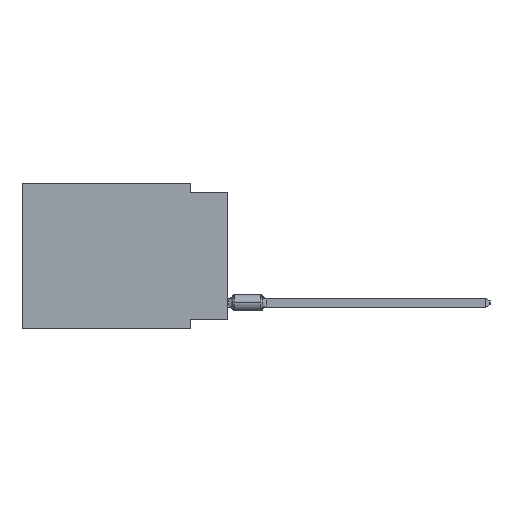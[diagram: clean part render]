
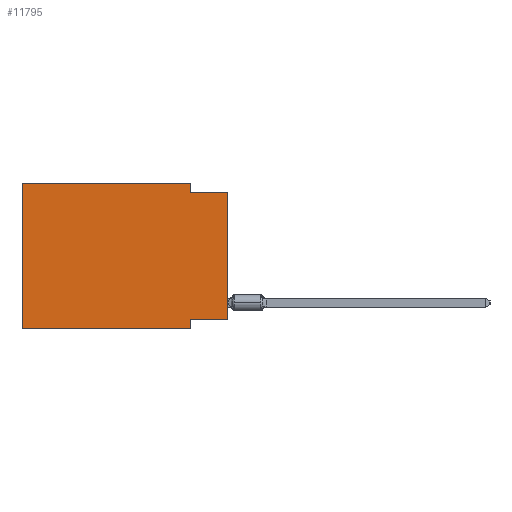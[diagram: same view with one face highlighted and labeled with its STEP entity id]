
A CAD part, left-side view. The second image highlights one B-rep face of the part: STEP entity #11795.
In plain terms, the highlighted planar face has unit normal (-1, 0, 0).
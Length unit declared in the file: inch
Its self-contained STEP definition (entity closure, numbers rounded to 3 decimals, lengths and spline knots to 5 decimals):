
#186 = VECTOR ( 'NONE', #24323, 39.37008 ) ;
#925 = ORIENTED_EDGE ( 'NONE', *, *, #29303, .F. ) ;
#1078 = DIRECTION ( 'NONE',  ( 0., 0., 1. ) ) ;
#1138 = VERTEX_POINT ( 'NONE', #26787 ) ;
#2114 = EDGE_CURVE ( 'NONE', #17205, #2430, #9782, .T. ) ;
#2336 = CARTESIAN_POINT ( 'NONE',  ( 0., 0.1, -0.365 ) ) ;
#2430 = VERTEX_POINT ( 'NONE', #2944 ) ;
#2562 = ORIENTED_EDGE ( 'NONE', *, *, #2114, .T. ) ;
#2828 = DIRECTION ( 'NONE',  ( 0., 1., 0. ) ) ;
#2858 = CARTESIAN_POINT ( 'NONE',  ( 0., 0.1, 0. ) ) ;
#2944 = CARTESIAN_POINT ( 'NONE',  ( 0., 0., -0.025 ) ) ;
#3008 = CARTESIAN_POINT ( 'NONE',  ( 0., 0., -0.365 ) ) ;
#3249 = DIRECTION ( 'NONE',  ( 0., 0., -1. ) ) ;
#4043 = LINE ( 'NONE', #18468, #186 ) ;
#4819 = CARTESIAN_POINT ( 'NONE',  ( 0., 0.55, -0.39 ) ) ;
#6089 = EDGE_CURVE ( 'NONE', #13038, #1138, #30358, .T. ) ;
#8978 = DIRECTION ( 'NONE',  ( 0., -1., 0. ) ) ;
#9512 = VERTEX_POINT ( 'NONE', #4819 ) ;
#9751 = EDGE_CURVE ( 'NONE', #30441, #13185, #4043, .T. ) ;
#9782 = LINE ( 'NONE', #32372, #20510 ) ;
#10248 = CARTESIAN_POINT ( 'NONE',  ( 0., 0.1, 0. ) ) ;
#11617 = CARTESIAN_POINT ( 'NONE',  ( 0., 0., -0.025 ) ) ;
#11773 = PLANE ( 'NONE',  #33305 ) ;
#11795 = ADVANCED_FACE ( 'NONE', ( #17851 ), #11773, .F. ) ;
#11846 = LINE ( 'NONE', #23409, #24939 ) ;
#12614 = EDGE_CURVE ( 'NONE', #9512, #17490, #23941, .T. ) ;
#13038 = VERTEX_POINT ( 'NONE', #2858 ) ;
#13185 = VERTEX_POINT ( 'NONE', #13442 ) ;
#13442 = CARTESIAN_POINT ( 'NONE',  ( 0., 0.1, -0.39 ) ) ;
#16122 = LINE ( 'NONE', #36368, #30781 ) ;
#17205 = VERTEX_POINT ( 'NONE', #35064 ) ;
#17490 = VERTEX_POINT ( 'NONE', #25002 ) ;
#17851 = FACE_OUTER_BOUND ( 'NONE', #36334, .T. ) ;
#18253 = CARTESIAN_POINT ( 'NONE',  ( 0., 0.55, 0. ) ) ;
#18468 = CARTESIAN_POINT ( 'NONE',  ( 0., 0.1, -0.39 ) ) ;
#19293 = VECTOR ( 'NONE', #2828, 39.37008 ) ;
#19436 = ORIENTED_EDGE ( 'NONE', *, *, #26586, .F. ) ;
#20510 = VECTOR ( 'NONE', #1078, 39.37008 ) ;
#20993 = ORIENTED_EDGE ( 'NONE', *, *, #9751, .F. ) ;
#22398 = VECTOR ( 'NONE', #35484, 39.37008 ) ;
#22407 = ORIENTED_EDGE ( 'NONE', *, *, #6089, .F. ) ;
#23381 = LINE ( 'NONE', #11617, #27412 ) ;
#23409 = CARTESIAN_POINT ( 'NONE',  ( 0., 0.55, 0. ) ) ;
#23941 = LINE ( 'NONE', #18253, #22398 ) ;
#24119 = DIRECTION ( 'NONE',  ( 0., 0., -1. ) ) ;
#24323 = DIRECTION ( 'NONE',  ( 0., 0., -1. ) ) ;
#24449 = VECTOR ( 'NONE', #24119, 39.37008 ) ;
#24939 = VECTOR ( 'NONE', #8978, 39.37008 ) ;
#25002 = CARTESIAN_POINT ( 'NONE',  ( 0., 0.55, 0. ) ) ;
#26347 = LINE ( 'NONE', #3008, #19293 ) ;
#26586 = EDGE_CURVE ( 'NONE', #17490, #13038, #11846, .T. ) ;
#26787 = CARTESIAN_POINT ( 'NONE',  ( 0., 0.1, -0.025 ) ) ;
#27412 = VECTOR ( 'NONE', #37012, 39.37008 ) ;
#29146 = ORIENTED_EDGE ( 'NONE', *, *, #34844, .F. ) ;
#29303 = EDGE_CURVE ( 'NONE', #1138, #2430, #23381, .T. ) ;
#30214 = ORIENTED_EDGE ( 'NONE', *, *, #34680, .T. ) ;
#30358 = LINE ( 'NONE', #10248, #24449 ) ;
#30441 = VERTEX_POINT ( 'NONE', #2336 ) ;
#30781 = VECTOR ( 'NONE', #36749, 39.37008 ) ;
#31370 = ORIENTED_EDGE ( 'NONE', *, *, #12614, .F. ) ;
#32036 = CARTESIAN_POINT ( 'NONE',  ( 0., 0.55, 0. ) ) ;
#32372 = CARTESIAN_POINT ( 'NONE',  ( 0., 0., 0. ) ) ;
#33305 = AXIS2_PLACEMENT_3D ( 'NONE', #32036, #34508, #3249 ) ;
#34508 = DIRECTION ( 'NONE',  ( 1., 0., 0. ) ) ;
#34680 = EDGE_CURVE ( 'NONE', #9512, #13185, #16122, .T. ) ;
#34844 = EDGE_CURVE ( 'NONE', #17205, #30441, #26347, .T. ) ;
#35064 = CARTESIAN_POINT ( 'NONE',  ( 0., 0., -0.365 ) ) ;
#35484 = DIRECTION ( 'NONE',  ( 0., 0., 1. ) ) ;
#36334 = EDGE_LOOP ( 'NONE', ( #2562, #925, #22407, #19436, #31370, #30214, #20993, #29146 ) ) ;
#36368 = CARTESIAN_POINT ( 'NONE',  ( 0., 0.55, -0.39 ) ) ;
#36749 = DIRECTION ( 'NONE',  ( 0., -1., 0. ) ) ;
#37012 = DIRECTION ( 'NONE',  ( 0., -1., 0. ) ) ;
